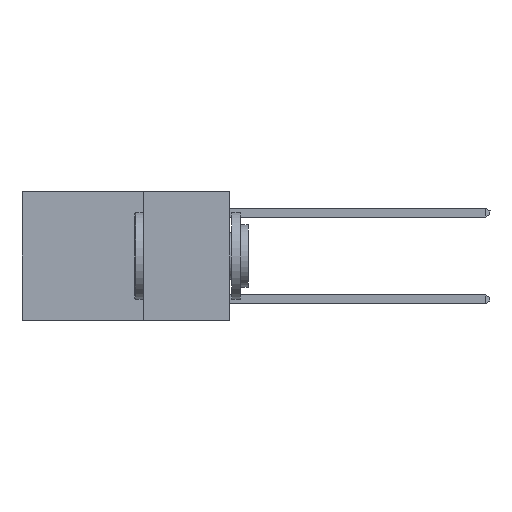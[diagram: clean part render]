
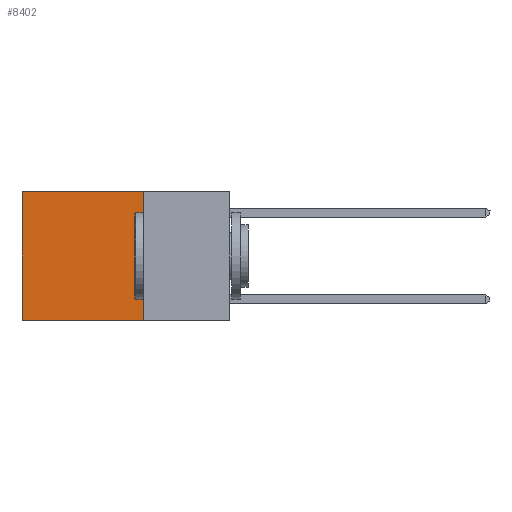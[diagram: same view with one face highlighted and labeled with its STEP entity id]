
A CAD part, left-side view. The second image highlights one B-rep face of the part: STEP entity #8402.
In plain terms, the highlighted planar face has unit normal (-1, 0, 0).
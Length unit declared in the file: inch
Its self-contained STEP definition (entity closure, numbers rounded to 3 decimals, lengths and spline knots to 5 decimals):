
#305 = CARTESIAN_POINT ( 'NONE',  ( 0.2625, 0.6, 0. ) ) ;
#432 = VECTOR ( 'NONE', #5336, 39.37008 ) ;
#1036 = FACE_OUTER_BOUND ( 'NONE', #6780, .T. ) ;
#1109 = CARTESIAN_POINT ( 'NONE',  ( 0.2625, 0.25, 0. ) ) ;
#1798 = VECTOR ( 'NONE', #5864, 39.37008 ) ;
#1807 = ORIENTED_EDGE ( 'NONE', *, *, #9151, .T. ) ;
#2400 = DIRECTION ( 'NONE',  ( 0., 0., -1. ) ) ;
#2481 = CARTESIAN_POINT ( 'NONE',  ( 0.2625, 0.6, 0. ) ) ;
#3290 = VERTEX_POINT ( 'NONE', #305 ) ;
#3699 = VECTOR ( 'NONE', #9827, 39.37008 ) ;
#3835 = CARTESIAN_POINT ( 'NONE',  ( 0.2625, 0.25, -0.37 ) ) ;
#3939 = VERTEX_POINT ( 'NONE', #4695 ) ;
#3974 = CARTESIAN_POINT ( 'NONE',  ( 0.2625, 0.6, -0.37 ) ) ;
#4695 = CARTESIAN_POINT ( 'NONE',  ( 0.2625, 0.25, 0. ) ) ;
#5325 = ORIENTED_EDGE ( 'NONE', *, *, #12936, .T. ) ;
#5336 = DIRECTION ( 'NONE',  ( 0., 1., 0. ) ) ;
#5461 = DIRECTION ( 'NONE',  ( 1., 0., 0. ) ) ;
#5864 = DIRECTION ( 'NONE',  ( 0., 1., 0. ) ) ;
#6577 = LINE ( 'NONE', #2481, #7226 ) ;
#6780 = EDGE_LOOP ( 'NONE', ( #5325, #9831, #12212, #1807 ) ) ;
#7226 = VECTOR ( 'NONE', #10940, 39.37008 ) ;
#7554 = CARTESIAN_POINT ( 'NONE',  ( 0.2625, 0.25, 0. ) ) ;
#7713 = AXIS2_PLACEMENT_3D ( 'NONE', #1109, #5461, #2400 ) ;
#8345 = EDGE_CURVE ( 'NONE', #3939, #11538, #10988, .T. ) ;
#8402 = ADVANCED_FACE ( 'NONE', ( #1036 ), #12063, .F. ) ;
#9151 = EDGE_CURVE ( 'NONE', #3939, #3290, #11543, .T. ) ;
#9827 = DIRECTION ( 'NONE',  ( 0., 0., -1. ) ) ;
#9831 = ORIENTED_EDGE ( 'NONE', *, *, #12715, .F. ) ;
#10940 = DIRECTION ( 'NONE',  ( 0., 0., -1. ) ) ;
#10988 = LINE ( 'NONE', #7554, #3699 ) ;
#11263 = CARTESIAN_POINT ( 'NONE',  ( 0.2625, 0.25, 0. ) ) ;
#11283 = LINE ( 'NONE', #3835, #1798 ) ;
#11538 = VERTEX_POINT ( 'NONE', #12207 ) ;
#11543 = LINE ( 'NONE', #11263, #432 ) ;
#12063 = PLANE ( 'NONE',  #7713 ) ;
#12207 = CARTESIAN_POINT ( 'NONE',  ( 0.2625, 0.25, -0.37 ) ) ;
#12212 = ORIENTED_EDGE ( 'NONE', *, *, #8345, .F. ) ;
#12715 = EDGE_CURVE ( 'NONE', #11538, #13648, #11283, .T. ) ;
#12936 = EDGE_CURVE ( 'NONE', #3290, #13648, #6577, .T. ) ;
#13648 = VERTEX_POINT ( 'NONE', #3974 ) ;
